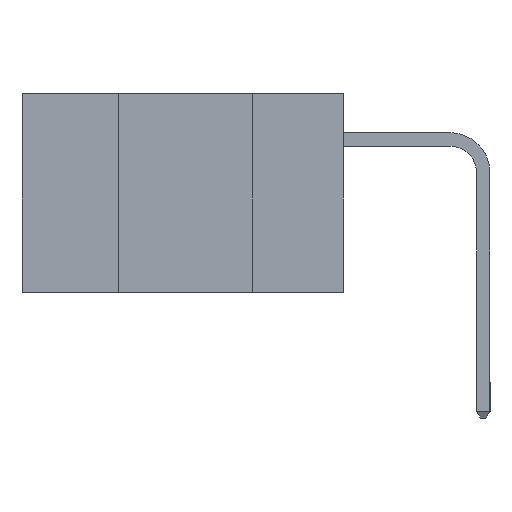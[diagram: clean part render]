
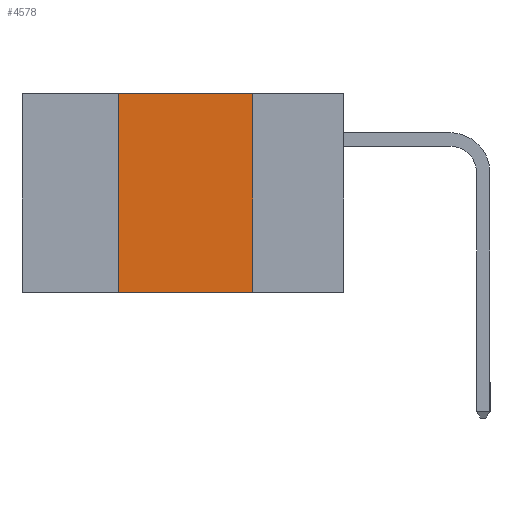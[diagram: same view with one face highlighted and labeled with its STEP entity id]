
A CAD part, left-side view. The second image highlights one B-rep face of the part: STEP entity #4578.
In plain terms, the highlighted planar face has unit normal (-1, 0, 0).
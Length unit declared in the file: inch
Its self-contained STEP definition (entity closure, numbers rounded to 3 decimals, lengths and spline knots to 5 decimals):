
#1521 = EDGE_CURVE ( 'NONE', #6700, #24982, #24166, .T. ) ;
#2051 = ORIENTED_EDGE ( 'NONE', *, *, #1521, .T. ) ;
#3604 = ORIENTED_EDGE ( 'NONE', *, *, #18042, .F. ) ;
#3713 = EDGE_CURVE ( 'NONE', #7051, #24982, #17829, .T. ) ;
#4578 = ADVANCED_FACE ( 'NONE', ( #23816 ), #16164, .F. ) ;
#4988 = LINE ( 'NONE', #20246, #15288 ) ;
#5070 = CARTESIAN_POINT ( 'NONE',  ( 0., 0.17, -0.37 ) ) ;
#5857 = DIRECTION ( 'NONE',  ( 0., 0., 1. ) ) ;
#6027 = CARTESIAN_POINT ( 'NONE',  ( 0., 0.17, 0. ) ) ;
#6700 = VERTEX_POINT ( 'NONE', #19149 ) ;
#7051 = VERTEX_POINT ( 'NONE', #13915 ) ;
#7484 = EDGE_CURVE ( 'NONE', #25779, #7051, #10529, .T. ) ;
#9994 = DIRECTION ( 'NONE',  ( 0., 0., -1. ) ) ;
#10529 = LINE ( 'NONE', #18405, #26147 ) ;
#12227 = DIRECTION ( 'NONE',  ( 0., -1., 0. ) ) ;
#12410 = DIRECTION ( 'NONE',  ( 0., 0., -1. ) ) ;
#13307 = VECTOR ( 'NONE', #21073, 39.37008 ) ;
#13597 = CARTESIAN_POINT ( 'NONE',  ( 0., 0.42, 0. ) ) ;
#13915 = CARTESIAN_POINT ( 'NONE',  ( 0., 0.17, 0. ) ) ;
#13919 = CARTESIAN_POINT ( 'NONE',  ( 0., 0.6, -0.37 ) ) ;
#14320 = DIRECTION ( 'NONE',  ( 1., 0., 0. ) ) ;
#14585 = ORIENTED_EDGE ( 'NONE', *, *, #3713, .F. ) ;
#15287 = AXIS2_PLACEMENT_3D ( 'NONE', #22374, #14320, #9994 ) ;
#15288 = VECTOR ( 'NONE', #5857, 39.37008 ) ;
#16164 = PLANE ( 'NONE',  #15287 ) ;
#17829 = LINE ( 'NONE', #6027, #23219 ) ;
#18042 = EDGE_CURVE ( 'NONE', #6700, #25779, #4988, .T. ) ;
#18405 = CARTESIAN_POINT ( 'NONE',  ( 0., 0.6, 0. ) ) ;
#19149 = CARTESIAN_POINT ( 'NONE',  ( 0., 0.42, -0.37 ) ) ;
#20246 = CARTESIAN_POINT ( 'NONE',  ( 0., 0.42, 0. ) ) ;
#21073 = DIRECTION ( 'NONE',  ( 0., -1., 0. ) ) ;
#22374 = CARTESIAN_POINT ( 'NONE',  ( 0., 0.6, 0. ) ) ;
#23219 = VECTOR ( 'NONE', #12410, 39.37008 ) ;
#23816 = FACE_OUTER_BOUND ( 'NONE', #25689, .T. ) ;
#24166 = LINE ( 'NONE', #13919, #13307 ) ;
#24982 = VERTEX_POINT ( 'NONE', #5070 ) ;
#25689 = EDGE_LOOP ( 'NONE', ( #14585, #25694, #3604, #2051 ) ) ;
#25694 = ORIENTED_EDGE ( 'NONE', *, *, #7484, .F. ) ;
#25779 = VERTEX_POINT ( 'NONE', #13597 ) ;
#26147 = VECTOR ( 'NONE', #12227, 39.37008 ) ;
